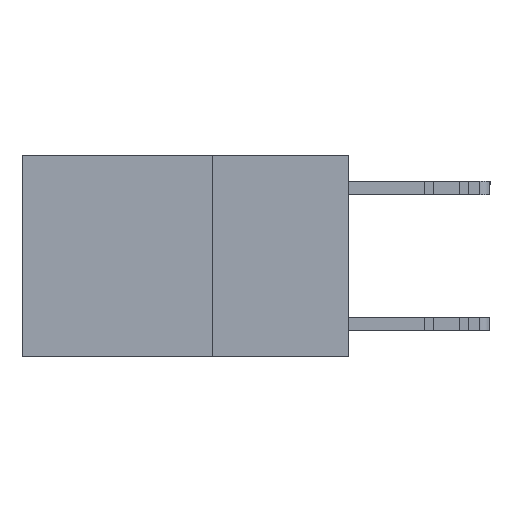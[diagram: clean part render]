
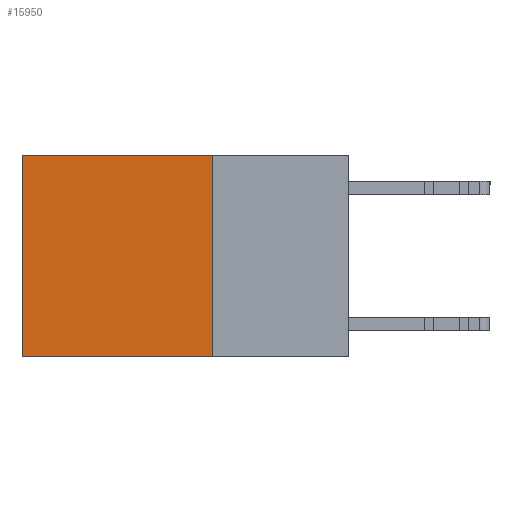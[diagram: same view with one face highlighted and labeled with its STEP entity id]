
A CAD part, left-side view. The second image highlights one B-rep face of the part: STEP entity #15950.
In plain terms, the highlighted planar face has unit normal (-1, 0, 0).
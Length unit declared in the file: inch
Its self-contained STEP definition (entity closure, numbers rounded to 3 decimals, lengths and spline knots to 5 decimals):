
#45 = ORIENTED_EDGE ( 'NONE', *, *, #1862, .F. ) ;
#130 = FACE_OUTER_BOUND ( 'NONE', #2041, .T. ) ;
#206 = VECTOR ( 'NONE', #12333, 39.37008 ) ;
#239 = LINE ( 'NONE', #21936, #6055 ) ;
#1862 = EDGE_CURVE ( 'NONE', #15397, #5559, #2614, .T. ) ;
#2041 = EDGE_LOOP ( 'NONE', ( #25266, #29537, #45, #5637 ) ) ;
#2614 = LINE ( 'NONE', #27014, #206 ) ;
#5559 = VERTEX_POINT ( 'NONE', #26915 ) ;
#5637 = ORIENTED_EDGE ( 'NONE', *, *, #21192, .T. ) ;
#6055 = VECTOR ( 'NONE', #19538, 39.37008 ) ;
#6713 = CARTESIAN_POINT ( 'NONE',  ( 0.2625, 0.25, 0. ) ) ;
#7442 = CARTESIAN_POINT ( 'NONE',  ( 0.2625, 0.6, -0.37 ) ) ;
#7520 = LINE ( 'NONE', #14086, #16869 ) ;
#8714 = VERTEX_POINT ( 'NONE', #7442 ) ;
#9851 = PLANE ( 'NONE',  #10317 ) ;
#10317 = AXIS2_PLACEMENT_3D ( 'NONE', #14359, #24078, #21386 ) ;
#12333 = DIRECTION ( 'NONE',  ( 0., 0., -1. ) ) ;
#13017 = VECTOR ( 'NONE', #26159, 39.37008 ) ;
#14086 = CARTESIAN_POINT ( 'NONE',  ( 0.2625, 0.6, 0. ) ) ;
#14195 = EDGE_CURVE ( 'NONE', #27907, #8714, #7520, .T. ) ;
#14251 = CARTESIAN_POINT ( 'NONE',  ( 0.2625, 0.25, 0. ) ) ;
#14359 = CARTESIAN_POINT ( 'NONE',  ( 0.2625, 0.25, 0. ) ) ;
#15397 = VERTEX_POINT ( 'NONE', #14251 ) ;
#15950 = ADVANCED_FACE ( 'NONE', ( #130 ), #9851, .F. ) ;
#16211 = CARTESIAN_POINT ( 'NONE',  ( 0.2625, 0.6, 0. ) ) ;
#16869 = VECTOR ( 'NONE', #23817, 39.37008 ) ;
#18819 = LINE ( 'NONE', #6713, #13017 ) ;
#19538 = DIRECTION ( 'NONE',  ( 0., 1., 0. ) ) ;
#21192 = EDGE_CURVE ( 'NONE', #15397, #27907, #18819, .T. ) ;
#21386 = DIRECTION ( 'NONE',  ( 0., 0., -1. ) ) ;
#21936 = CARTESIAN_POINT ( 'NONE',  ( 0.2625, 0.25, -0.37 ) ) ;
#23817 = DIRECTION ( 'NONE',  ( 0., 0., -1. ) ) ;
#24078 = DIRECTION ( 'NONE',  ( 1., 0., 0. ) ) ;
#25266 = ORIENTED_EDGE ( 'NONE', *, *, #14195, .T. ) ;
#26159 = DIRECTION ( 'NONE',  ( 0., 1., 0. ) ) ;
#26420 = EDGE_CURVE ( 'NONE', #5559, #8714, #239, .T. ) ;
#26915 = CARTESIAN_POINT ( 'NONE',  ( 0.2625, 0.25, -0.37 ) ) ;
#27014 = CARTESIAN_POINT ( 'NONE',  ( 0.2625, 0.25, 0. ) ) ;
#27907 = VERTEX_POINT ( 'NONE', #16211 ) ;
#29537 = ORIENTED_EDGE ( 'NONE', *, *, #26420, .F. ) ;
